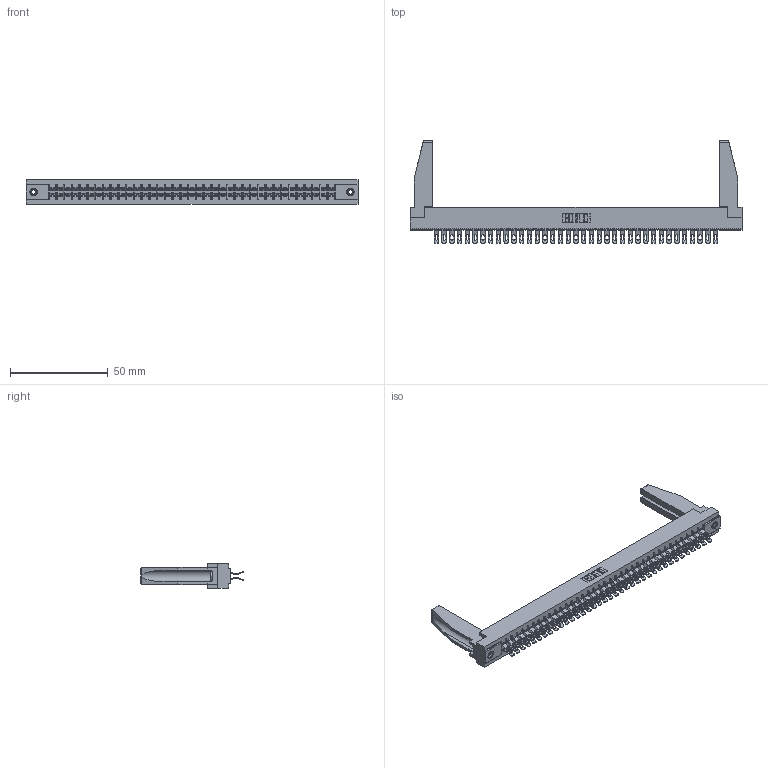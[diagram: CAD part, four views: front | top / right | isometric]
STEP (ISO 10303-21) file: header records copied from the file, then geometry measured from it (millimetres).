
FILE_DESCRIPTION (( 'STEP AP203' ), '1' );
FILE_NAME ('315-074-555-278.STEP', '2019-09-10T22:14:26', ( '' ), ( '' ), 'SwSTEP 2.0', 'SolidWorks 2016', '' );
FILE_SCHEMA (( 'CONFIG_CONTROL_DESIGN' ));
Length unit declared in the file: inch
Products named in the file (5): 305 Part_.156 Dia; 305-290-001_555; 345-250-001_345-250-001-102; 307-220-078; 315-074-555-278
Assembly tree (79 placements, depth 2):
  315-074-555-278
    305 Part_.156 Dia
    305-290-001_555  x74
    345-250-001_345-250-001-102  x2
    307-220-078  x2
Bounding box: 169.62 x 52.45 x 12.7 mm (x, y, z)
Volume: 21879.7 mm3; surface area: 27855.3 mm2
Topology: 79 solids, 79 shells, 5130 faces, 15261 edges, 9966 vertices
Faces by surface type: plane 2520, cylinder 2446, sphere 148, cone 12, torus 4
Entity records: 43733 total; most frequent: CARTESIAN_POINT 7261, ORIENTED_EDGE 7156, DIRECTION 6980, EDGE_CURVE 3578, LINE 2866, VECTOR 2866, VERTEX_POINT 2280, AXIS2_PLACEMENT_3D 2057
